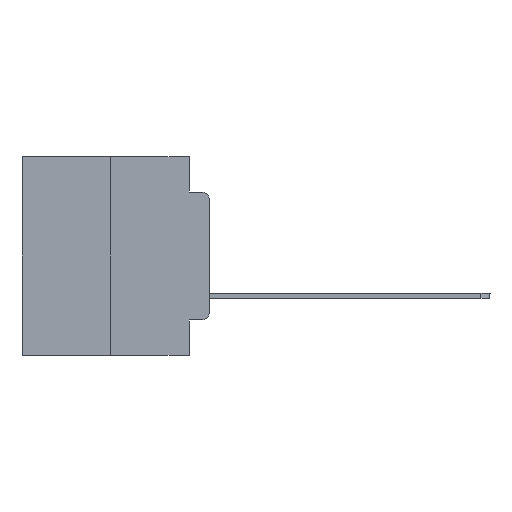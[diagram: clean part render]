
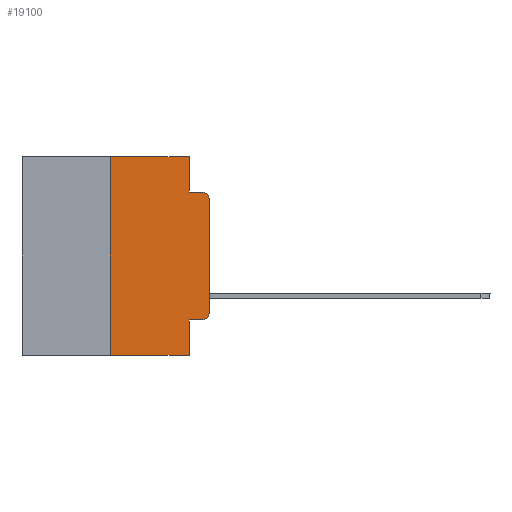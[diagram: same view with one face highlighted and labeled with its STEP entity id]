
A CAD part, left-side view. The second image highlights one B-rep face of the part: STEP entity #19100.
In plain terms, the highlighted planar face has unit normal (-1, 0, 0).
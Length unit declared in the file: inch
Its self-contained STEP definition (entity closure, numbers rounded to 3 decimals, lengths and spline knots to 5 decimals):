
#487 = VERTEX_POINT ( 'NONE', #24673 ) ;
#952 = DIRECTION ( 'NONE',  ( 0., -1., 0. ) ) ;
#1104 = CARTESIAN_POINT ( 'NONE',  ( 0., 0.25, -0.5 ) ) ;
#1335 = LINE ( 'NONE', #19071, #17948 ) ;
#1799 = CARTESIAN_POINT ( 'NONE',  ( 0., 0.473, 0. ) ) ;
#2438 = LINE ( 'NONE', #24786, #24233 ) ;
#2626 = CARTESIAN_POINT ( 'NONE',  ( 0., 0.051, 0. ) ) ;
#2706 = DIRECTION ( 'NONE',  ( 0., 0., 1. ) ) ;
#3421 = VECTOR ( 'NONE', #22344, 39.37008 ) ;
#3947 = EDGE_CURVE ( 'NONE', #7082, #16911, #24319, .T. ) ;
#4396 = CARTESIAN_POINT ( 'NONE',  ( 0., 0.25, 0. ) ) ;
#4465 = CARTESIAN_POINT ( 'NONE',  ( 0., 0.051, 0. ) ) ;
#4781 = EDGE_CURVE ( 'NONE', #20989, #11584, #1335, .T. ) ;
#5238 = CARTESIAN_POINT ( 'NONE',  ( 0., 0.473, 0. ) ) ;
#5930 = PLANE ( 'NONE',  #20743 ) ;
#6239 = CARTESIAN_POINT ( 'NONE',  ( 0., 0.051, -0.4115 ) ) ;
#6353 = LINE ( 'NONE', #2626, #13011 ) ;
#6428 = VECTOR ( 'NONE', #7277, 39.37008 ) ;
#7082 = VERTEX_POINT ( 'NONE', #11296 ) ;
#7277 = DIRECTION ( 'NONE',  ( 0., 0., 1. ) ) ;
#7902 = DIRECTION ( 'NONE',  ( 0., 0., -1. ) ) ;
#7909 = ORIENTED_EDGE ( 'NONE', *, *, #24430, .T. ) ;
#7986 = EDGE_CURVE ( 'NONE', #7082, #13892, #24533, .T. ) ;
#8102 = VERTEX_POINT ( 'NONE', #14668 ) ;
#8547 = VERTEX_POINT ( 'NONE', #1104 ) ;
#8767 = VERTEX_POINT ( 'NONE', #15659 ) ;
#8882 = LINE ( 'NONE', #13099, #6428 ) ;
#9083 = CIRCLE ( 'NONE', #25113, 0.02 ) ;
#9213 = ORIENTED_EDGE ( 'NONE', *, *, #7986, .F. ) ;
#10395 = DIRECTION ( 'NONE',  ( 0., -1., 0. ) ) ;
#10587 = CARTESIAN_POINT ( 'NONE',  ( 0., 0.02, -0.1085 ) ) ;
#10859 = EDGE_CURVE ( 'NONE', #8547, #13892, #2438, .T. ) ;
#11296 = CARTESIAN_POINT ( 'NONE',  ( 0., 0.051, -0.4115 ) ) ;
#11584 = VERTEX_POINT ( 'NONE', #16821 ) ;
#11838 = CARTESIAN_POINT ( 'NONE',  ( 0., 0.02, -0.3915 ) ) ;
#12153 = ORIENTED_EDGE ( 'NONE', *, *, #23786, .T. ) ;
#12238 = DIRECTION ( 'NONE',  ( 0., 0., -1. ) ) ;
#12448 = CIRCLE ( 'NONE', #18779, 0.02 ) ;
#12524 = CARTESIAN_POINT ( 'NONE',  ( 0., 0.051, -0.0885 ) ) ;
#13011 = VECTOR ( 'NONE', #18510, 39.37008 ) ;
#13099 = CARTESIAN_POINT ( 'NONE',  ( 0., 0., 0. ) ) ;
#13502 = VECTOR ( 'NONE', #19656, 39.37008 ) ;
#13698 = LINE ( 'NONE', #5238, #13502 ) ;
#13892 = VERTEX_POINT ( 'NONE', #25789 ) ;
#14092 = ORIENTED_EDGE ( 'NONE', *, *, #21431, .T. ) ;
#14383 = DIRECTION ( 'NONE',  ( 1., 0., 0. ) ) ;
#14456 = ORIENTED_EDGE ( 'NONE', *, *, #14494, .F. ) ;
#14494 = EDGE_CURVE ( 'NONE', #8102, #20989, #6353, .T. ) ;
#14668 = CARTESIAN_POINT ( 'NONE',  ( 0., 0.051, 0. ) ) ;
#14772 = CARTESIAN_POINT ( 'NONE',  ( 0., 0.25, 0. ) ) ;
#15146 = VERTEX_POINT ( 'NONE', #4396 ) ;
#15659 = CARTESIAN_POINT ( 'NONE',  ( 0., 0., -0.1085 ) ) ;
#16368 = FACE_OUTER_BOUND ( 'NONE', #18411, .T. ) ;
#16478 = VECTOR ( 'NONE', #16632, 39.37008 ) ;
#16632 = DIRECTION ( 'NONE',  ( 0., 0., -1. ) ) ;
#16821 = CARTESIAN_POINT ( 'NONE',  ( 0., 0.02, -0.0885 ) ) ;
#16911 = VERTEX_POINT ( 'NONE', #22608 ) ;
#17048 = DIRECTION ( 'NONE',  ( -1., 0., 0. ) ) ;
#17668 = EDGE_CURVE ( 'NONE', #15146, #8102, #13698, .T. ) ;
#17921 = EDGE_CURVE ( 'NONE', #8547, #15146, #22683, .T. ) ;
#17948 = VECTOR ( 'NONE', #952, 39.37008 ) ;
#18411 = EDGE_LOOP ( 'NONE', ( #14092, #7909, #22298, #14456, #23891, #18957, #25609, #9213, #23829, #12153 ) ) ;
#18510 = DIRECTION ( 'NONE',  ( 0., 0., -1. ) ) ;
#18779 = AXIS2_PLACEMENT_3D ( 'NONE', #11838, #23710, #12238 ) ;
#18957 = ORIENTED_EDGE ( 'NONE', *, *, #17921, .F. ) ;
#19071 = CARTESIAN_POINT ( 'NONE',  ( 0., 0.051, -0.0885 ) ) ;
#19100 = ADVANCED_FACE ( 'NONE', ( #16368 ), #5930, .F. ) ;
#19656 = DIRECTION ( 'NONE',  ( 0., -1., 0. ) ) ;
#20296 = VECTOR ( 'NONE', #2706, 39.37008 ) ;
#20743 = AXIS2_PLACEMENT_3D ( 'NONE', #1799, #14383, #7902 ) ;
#20989 = VERTEX_POINT ( 'NONE', #12524 ) ;
#21431 = EDGE_CURVE ( 'NONE', #487, #8767, #8882, .T. ) ;
#22298 = ORIENTED_EDGE ( 'NONE', *, *, #4781, .F. ) ;
#22344 = DIRECTION ( 'NONE',  ( 0., -1., 0. ) ) ;
#22608 = CARTESIAN_POINT ( 'NONE',  ( 0., 0.02, -0.4115 ) ) ;
#22683 = LINE ( 'NONE', #14772, #20296 ) ;
#22735 = DIRECTION ( 'NONE',  ( 0., 0., -1. ) ) ;
#23710 = DIRECTION ( 'NONE',  ( -1., 0., 0. ) ) ;
#23786 = EDGE_CURVE ( 'NONE', #16911, #487, #12448, .T. ) ;
#23829 = ORIENTED_EDGE ( 'NONE', *, *, #3947, .T. ) ;
#23891 = ORIENTED_EDGE ( 'NONE', *, *, #17668, .F. ) ;
#24233 = VECTOR ( 'NONE', #10395, 39.37008 ) ;
#24319 = LINE ( 'NONE', #6239, #3421 ) ;
#24430 = EDGE_CURVE ( 'NONE', #8767, #11584, #9083, .T. ) ;
#24533 = LINE ( 'NONE', #4465, #16478 ) ;
#24673 = CARTESIAN_POINT ( 'NONE',  ( 0., 0., -0.3915 ) ) ;
#24786 = CARTESIAN_POINT ( 'NONE',  ( 0., 0.473, -0.5 ) ) ;
#25113 = AXIS2_PLACEMENT_3D ( 'NONE', #10587, #17048, #22735 ) ;
#25609 = ORIENTED_EDGE ( 'NONE', *, *, #10859, .T. ) ;
#25789 = CARTESIAN_POINT ( 'NONE',  ( 0., 0.051, -0.5 ) ) ;
